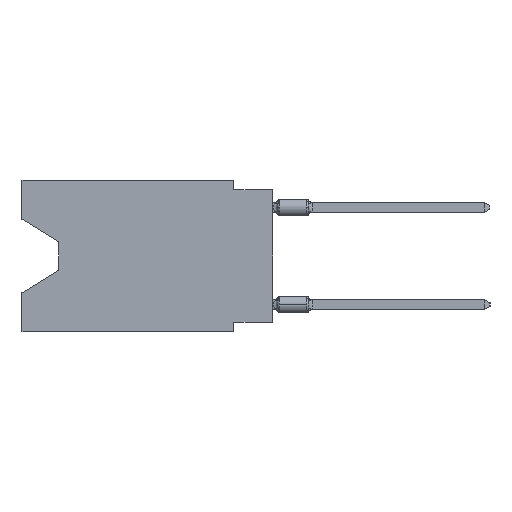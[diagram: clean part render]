
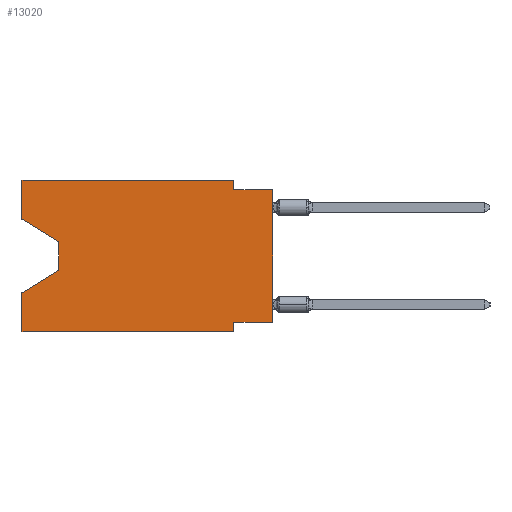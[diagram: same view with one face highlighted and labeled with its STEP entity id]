
A CAD part, left-side view. The second image highlights one B-rep face of the part: STEP entity #13020.
In plain terms, the highlighted planar face has unit normal (-1, 0, 0).
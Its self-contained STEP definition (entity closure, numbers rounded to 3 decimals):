
#81 = DIRECTION ( 'NONE',  ( 0., 0., -1. ) ) ;
#1375 = CARTESIAN_POINT ( 'NONE',  ( 0., 16.383, 0. ) ) ;
#2027 = VECTOR ( 'NONE', #14716, 1000. ) ;
#2870 = LINE ( 'NONE', #36767, #34036 ) ;
#2876 = VECTOR ( 'NONE', #17713, 1000. ) ;
#2942 = VECTOR ( 'NONE', #22176, 1000. ) ;
#3077 = CARTESIAN_POINT ( 'NONE',  ( 0., 2.54, -9.906 ) ) ;
#3253 = EDGE_CURVE ( 'NONE', #7440, #22416, #24430, .T. ) ;
#3357 = EDGE_CURVE ( 'NONE', #4539, #31676, #18509, .T. ) ;
#3481 = DIRECTION ( 'NONE',  ( 0., 0., 1. ) ) ;
#3754 = CARTESIAN_POINT ( 'NONE',  ( 0., 16.383, -7.36 ) ) ;
#4098 = DIRECTION ( 'NONE',  ( 0., 0.855, -0.519 ) ) ;
#4539 = VERTEX_POINT ( 'NONE', #7334 ) ;
#4656 = LINE ( 'NONE', #21790, #8006 ) ;
#5858 = ORIENTED_EDGE ( 'NONE', *, *, #3357, .F. ) ;
#5873 = CARTESIAN_POINT ( 'NONE',  ( 0., 0., -9.271 ) ) ;
#6345 = CARTESIAN_POINT ( 'NONE',  ( 0., 16.383, -2.546 ) ) ;
#6399 = DIRECTION ( 'NONE',  ( 0., 0., -1. ) ) ;
#7334 = CARTESIAN_POINT ( 'NONE',  ( 0., 16.383, 0. ) ) ;
#7440 = VERTEX_POINT ( 'NONE', #17113 ) ;
#7451 = CARTESIAN_POINT ( 'NONE',  ( 0., 13.97, -5.893 ) ) ;
#8006 = VECTOR ( 'NONE', #4098, 1000. ) ;
#8167 = EDGE_CURVE ( 'NONE', #18711, #33155, #16977, .T. ) ;
#8299 = EDGE_CURVE ( 'NONE', #23608, #22416, #11556, .T. ) ;
#8428 = ORIENTED_EDGE ( 'NONE', *, *, #11132, .F. ) ;
#9107 = DIRECTION ( 'NONE',  ( 0., 0., -1. ) ) ;
#9284 = VECTOR ( 'NONE', #26890, 1000. ) ;
#9578 = VERTEX_POINT ( 'NONE', #14692 ) ;
#9913 = PLANE ( 'NONE',  #33358 ) ;
#10236 = LINE ( 'NONE', #18447, #24233 ) ;
#10305 = VERTEX_POINT ( 'NONE', #16445 ) ;
#11132 = EDGE_CURVE ( 'NONE', #10305, #4539, #13976, .T. ) ;
#11556 = LINE ( 'NONE', #28516, #17512 ) ;
#12094 = VERTEX_POINT ( 'NONE', #3754 ) ;
#13020 = ADVANCED_FACE ( 'NONE', ( #31917 ), #9913, .F. ) ;
#13207 = CARTESIAN_POINT ( 'NONE',  ( 0., 2.54, -0.635 ) ) ;
#13240 = CARTESIAN_POINT ( 'NONE',  ( 0., 2.54, -9.906 ) ) ;
#13766 = CARTESIAN_POINT ( 'NONE',  ( 0., 16.383, -9.906 ) ) ;
#13901 = ORIENTED_EDGE ( 'NONE', *, *, #23583, .T. ) ;
#13913 = VECTOR ( 'NONE', #25048, 1000. ) ;
#13976 = LINE ( 'NONE', #22742, #2942 ) ;
#14191 = EDGE_CURVE ( 'NONE', #35449, #12094, #20790, .T. ) ;
#14692 = CARTESIAN_POINT ( 'NONE',  ( 0., 13.97, -4.013 ) ) ;
#14716 = DIRECTION ( 'NONE',  ( 0., 0., -1. ) ) ;
#15060 = LINE ( 'NONE', #34618, #27595 ) ;
#15686 = ORIENTED_EDGE ( 'NONE', *, *, #14191, .F. ) ;
#15808 = EDGE_CURVE ( 'NONE', #35449, #33155, #10236, .T. ) ;
#16445 = CARTESIAN_POINT ( 'NONE',  ( 0., 16.383, -2.546 ) ) ;
#16667 = ORIENTED_EDGE ( 'NONE', *, *, #8299, .F. ) ;
#16977 = LINE ( 'NONE', #13240, #2027 ) ;
#17113 = CARTESIAN_POINT ( 'NONE',  ( 0., 0., -9.271 ) ) ;
#17512 = VECTOR ( 'NONE', #31849, 1000. ) ;
#17713 = DIRECTION ( 'NONE',  ( 0., -0.855, -0.519 ) ) ;
#17717 = EDGE_CURVE ( 'NONE', #32570, #12094, #4656, .T. ) ;
#18447 = CARTESIAN_POINT ( 'NONE',  ( 0., 16.383, -9.906 ) ) ;
#18509 = LINE ( 'NONE', #1375, #9284 ) ;
#18711 = VERTEX_POINT ( 'NONE', #30616 ) ;
#18744 = ORIENTED_EDGE ( 'NONE', *, *, #8167, .F. ) ;
#19487 = ORIENTED_EDGE ( 'NONE', *, *, #30645, .F. ) ;
#20252 = CARTESIAN_POINT ( 'NONE',  ( 0., 16.383, 0. ) ) ;
#20790 = LINE ( 'NONE', #20252, #21281 ) ;
#21055 = DIRECTION ( 'NONE',  ( 0., -1., 0. ) ) ;
#21281 = VECTOR ( 'NONE', #3481, 1000. ) ;
#21545 = ORIENTED_EDGE ( 'NONE', *, *, #34520, .F. ) ;
#21790 = CARTESIAN_POINT ( 'NONE',  ( 0., 13.97, -5.893 ) ) ;
#22176 = DIRECTION ( 'NONE',  ( 0., 0., 1. ) ) ;
#22416 = VERTEX_POINT ( 'NONE', #27503 ) ;
#22742 = CARTESIAN_POINT ( 'NONE',  ( 0., 16.383, 0. ) ) ;
#22836 = ORIENTED_EDGE ( 'NONE', *, *, #15808, .T. ) ;
#22944 = LINE ( 'NONE', #6345, #2876 ) ;
#23583 = EDGE_CURVE ( 'NONE', #10305, #9578, #22944, .T. ) ;
#23608 = VERTEX_POINT ( 'NONE', #13207 ) ;
#24073 = CARTESIAN_POINT ( 'NONE',  ( 0., 0., 0. ) ) ;
#24233 = VECTOR ( 'NONE', #21055, 1000. ) ;
#24430 = LINE ( 'NONE', #24073, #36052 ) ;
#25048 = DIRECTION ( 'NONE',  ( 0., 1., 0. ) ) ;
#25824 = EDGE_LOOP ( 'NONE', ( #13901, #33399, #26173, #15686, #22836, #18744, #19487, #30944, #16667, #21545, #5858, #8428 ) ) ;
#26173 = ORIENTED_EDGE ( 'NONE', *, *, #17717, .T. ) ;
#26562 = CARTESIAN_POINT ( 'NONE',  ( 0., 2.54, 0. ) ) ;
#26890 = DIRECTION ( 'NONE',  ( 0., -1., 0. ) ) ;
#27503 = CARTESIAN_POINT ( 'NONE',  ( 0., 0., -0.635 ) ) ;
#27595 = VECTOR ( 'NONE', #9107, 1000. ) ;
#28516 = CARTESIAN_POINT ( 'NONE',  ( 0., 0., -0.635 ) ) ;
#30616 = CARTESIAN_POINT ( 'NONE',  ( 0., 2.54, -9.271 ) ) ;
#30645 = EDGE_CURVE ( 'NONE', #7440, #18711, #31373, .T. ) ;
#30944 = ORIENTED_EDGE ( 'NONE', *, *, #3253, .T. ) ;
#31373 = LINE ( 'NONE', #5873, #13913 ) ;
#31676 = VERTEX_POINT ( 'NONE', #26562 ) ;
#31849 = DIRECTION ( 'NONE',  ( 0., -1., 0. ) ) ;
#31917 = FACE_OUTER_BOUND ( 'NONE', #25824, .T. ) ;
#32098 = DIRECTION ( 'NONE',  ( 1., 0., 0. ) ) ;
#32570 = VERTEX_POINT ( 'NONE', #7451 ) ;
#33155 = VERTEX_POINT ( 'NONE', #3077 ) ;
#33358 = AXIS2_PLACEMENT_3D ( 'NONE', #35431, #32098, #6399 ) ;
#33399 = ORIENTED_EDGE ( 'NONE', *, *, #36785, .T. ) ;
#34036 = VECTOR ( 'NONE', #81, 1000. ) ;
#34520 = EDGE_CURVE ( 'NONE', #31676, #23608, #2870, .T. ) ;
#34618 = CARTESIAN_POINT ( 'NONE',  ( 0., 13.97, -4.013 ) ) ;
#35409 = DIRECTION ( 'NONE',  ( 0., 0., 1. ) ) ;
#35431 = CARTESIAN_POINT ( 'NONE',  ( 0., 16.383, 0. ) ) ;
#35449 = VERTEX_POINT ( 'NONE', #13766 ) ;
#36052 = VECTOR ( 'NONE', #35409, 1000. ) ;
#36767 = CARTESIAN_POINT ( 'NONE',  ( 0., 2.54, 0. ) ) ;
#36785 = EDGE_CURVE ( 'NONE', #9578, #32570, #15060, .T. ) ;
